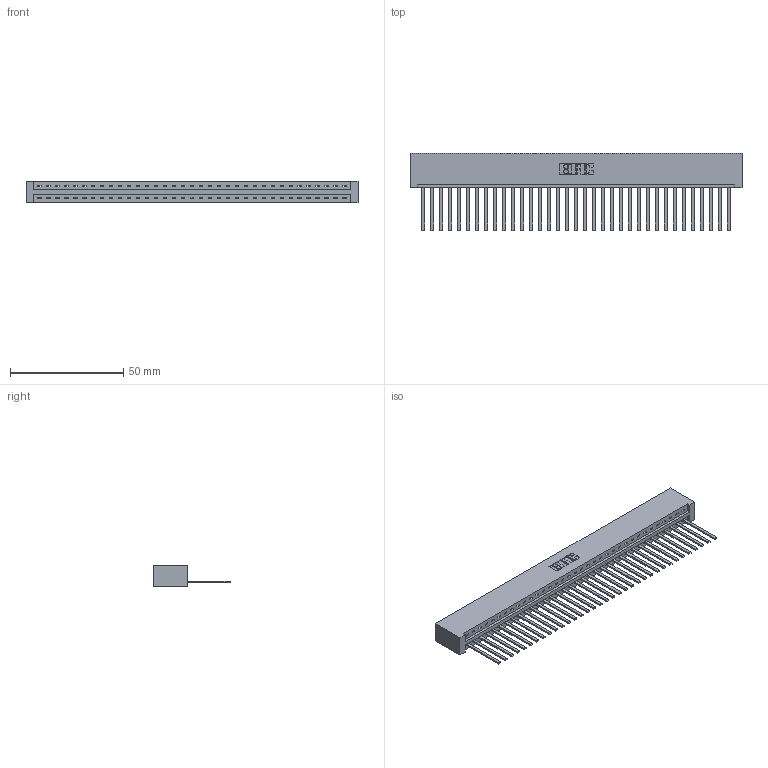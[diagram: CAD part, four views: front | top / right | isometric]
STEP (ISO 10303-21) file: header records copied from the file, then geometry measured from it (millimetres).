
FILE_DESCRIPTION (( 'STEP AP203' ), '1' );
FILE_NAME ('337-035-544-101.STEP', '2018-08-07T20:54:09', ( '' ), ( '' ), 'SwSTEP 2.0', 'SolidWorks 2016', '' );
FILE_SCHEMA (( 'CONFIG_CONTROL_DESIGN' ));
Length unit declared in the file: inch
Products named in the file (3): 337 Part_No Mounting Lugs; 345-292-001_345-293-144; 337-035-544-101
Assembly tree (36 placements, depth 2):
  337-035-544-101
    337 Part_No Mounting Lugs
    345-292-001_345-293-144  x35
Bounding box: 146.56 x 34.3 x 9.4 mm (x, y, z)
Volume: 16288.7 mm3; surface area: 18108 mm2
Topology: 36 solids, 36 shells, 2066 faces, 6237 edges, 4110 vertices
Faces by surface type: plane 1536, cylinder 530
Entity records: 26461 total; most frequent: CARTESIAN_POINT 4615, ORIENTED_EDGE 4586, DIRECTION 3887, EDGE_CURVE 2293, LINE 2177, VECTOR 2177, VERTEX_POINT 1526, AXIS2_PLACEMENT_3D 855
